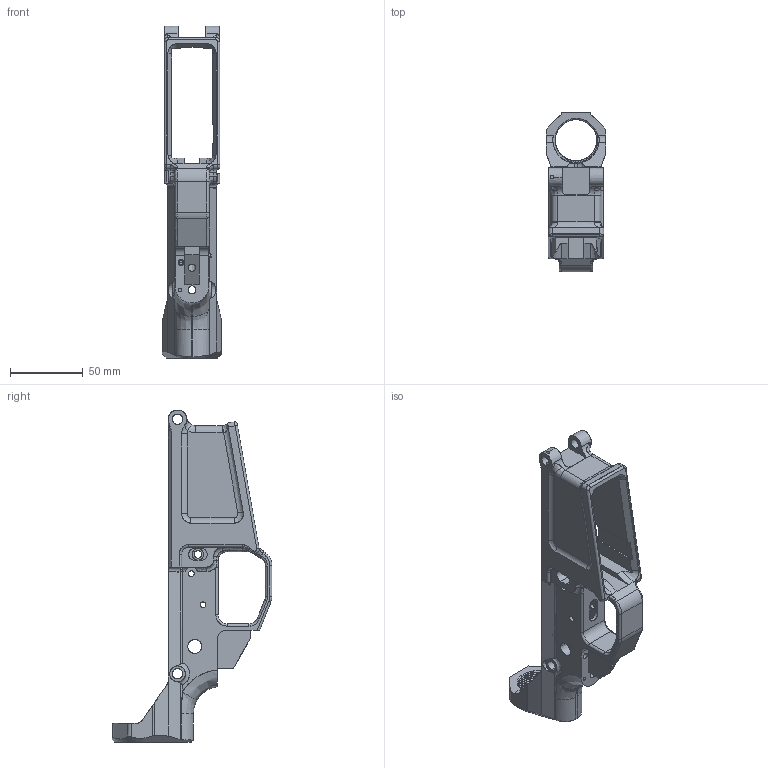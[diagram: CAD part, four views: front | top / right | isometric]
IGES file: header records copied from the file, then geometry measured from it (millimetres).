
Start section: SolidWorks IGES file using analytic representation for surfaces
Global section: file name: WX LOWER.IGS; native system: SolidWorks 2015; preprocessor: SolidWorks 2015; author: WarFairy; date: 160423.092321; units: inch
Bounding box: 40.64 x 109.71 x 227.84 mm (x, y, z)
Surface area: 62833.9 mm2 (no closed solid volume)
Topology: 0 solids, 0 shells, 445 faces, 6461 edges, 6456 vertices
Faces by surface type: bspline 236, revolution 209
